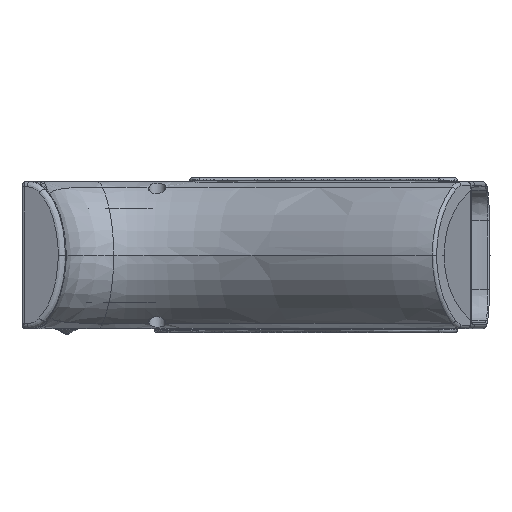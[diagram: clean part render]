
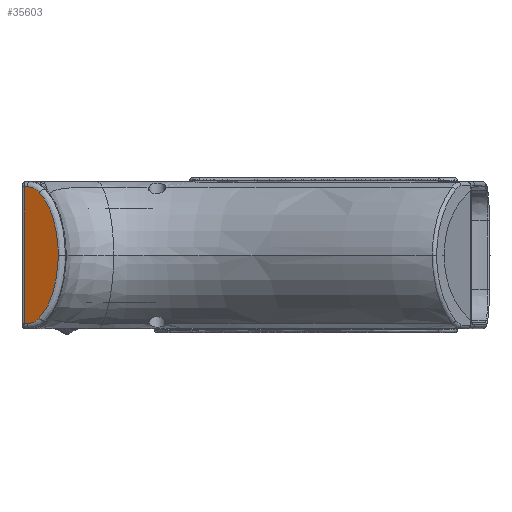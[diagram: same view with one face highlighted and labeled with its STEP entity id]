
A CAD part, left-side view. The second image highlights one B-rep face of the part: STEP entity #35603.
In plain terms, the highlighted planar face has unit normal (-0.906, 0.423, 0).
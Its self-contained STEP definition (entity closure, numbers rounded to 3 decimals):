
#2019=PLANE('',#37724);
#3836=FACE_OUTER_BOUND('',#5931,.T.);
#5931=EDGE_LOOP('',(#24339,#24340,#24341,#24342,#24343,#24344,#24345));
#8334=LINE('',#45406,#11125);
#8445=LINE('',#54969,#11236);
#8446=LINE('',#55000,#11237);
#11125=VECTOR('',#39023,1.);
#11236=VECTOR('',#39260,10.);
#11237=VECTOR('',#39261,1.);
#13998=B_SPLINE_CURVE_WITH_KNOTS('',3,(#54913,#54914,#54915,#54916,#54917,
#54918,#54919,#54920,#54921,#54922,#54923,#54924,#54925,#54926,#54927,#54928,
#54929,#54930,#54931,#54932,#54933,#54934,#54935,#54936,#54937),
 .UNSPECIFIED.,.F.,.F.,(4,2,2,2,2,2,2,2,2,1,2,2,4),(0.003,
0.144,0.288,0.431,0.573,0.714,
0.855,0.996,1.135,1.188,1.241,
1.293,1.332),.UNSPECIFIED.);
#13999=B_SPLINE_CURVE_WITH_KNOTS('',3,(#54963,#54964,#54965,#54966),
 .UNSPECIFIED.,.F.,.F.,(4,4),(-0.284,0.),.UNSPECIFIED.);
#14000=B_SPLINE_CURVE_WITH_KNOTS('',3,(#54971,#54972,#54973,#54974,#54975,
#54976,#54977,#54978,#54979,#54980,#54981,#54982,#54983,#54984,#54985,#54986,
#54987,#54988,#54989,#54990,#54991,#54992,#54993,#54994),.UNSPECIFIED.,
 .F.,.F.,(4,2,2,2,2,2,2,2,2,2,2,4),(0.197,0.236,0.287,
0.394,0.533,0.673,0.813,0.954,
1.096,1.239,1.383,1.523),
 .UNSPECIFIED.);
#14001=B_SPLINE_CURVE_WITH_KNOTS('',3,(#54996,#54997,#54998,#54999),
 .UNSPECIFIED.,.F.,.F.,(4,4),(-0.284,0.),.UNSPECIFIED.);
#14728=VERTEX_POINT('',#45401);
#14729=VERTEX_POINT('',#45404);
#14905=VERTEX_POINT('',#54460);
#14906=VERTEX_POINT('',#54912);
#14907=VERTEX_POINT('',#54968);
#14908=VERTEX_POINT('',#54970);
#14909=VERTEX_POINT('',#54995);
#18337=EDGE_CURVE('',#14729,#14728,#8334,.T.);
#18559=EDGE_CURVE('',#14905,#14906,#13998,.T.);
#18561=EDGE_CURVE('',#14906,#14729,#13999,.T.);
#18562=EDGE_CURVE('',#14728,#14907,#8445,.T.);
#18563=EDGE_CURVE('',#14908,#14905,#14000,.T.);
#18564=EDGE_CURVE('',#14909,#14908,#14001,.T.);
#18565=EDGE_CURVE('',#14907,#14909,#8446,.T.);
#24339=ORIENTED_EDGE('',*,*,#18562,.F.);
#24340=ORIENTED_EDGE('',*,*,#18337,.F.);
#24341=ORIENTED_EDGE('',*,*,#18561,.F.);
#24342=ORIENTED_EDGE('',*,*,#18559,.F.);
#24343=ORIENTED_EDGE('',*,*,#18563,.F.);
#24344=ORIENTED_EDGE('',*,*,#18564,.F.);
#24345=ORIENTED_EDGE('',*,*,#18565,.F.);
#35603=ADVANCED_FACE('',(#3836),#2019,.F.);
#37724=AXIS2_PLACEMENT_3D('',#54967,#39258,#39259);
#39023=DIRECTION('',(0.423,0.906,0.));
#39258=DIRECTION('center_axis',(0.906,-0.423,0.));
#39259=DIRECTION('ref_axis',(0.423,0.906,0.));
#39260=DIRECTION('',(0.,0.,1.));
#39261=DIRECTION('',(-0.423,-0.906,0.));
#45401=CARTESIAN_POINT('',(-0.852,-1.404,-13.4));
#45404=CARTESIAN_POINT('',(-1.16,-2.065,-13.4));
#45406=CARTESIAN_POINT('',(-5.081,-10.474,-13.4));
#54460=CARTESIAN_POINT('',(-3.998,-8.151,0.));
#54912=CARTESIAN_POINT('',(-2.228,-4.355,-12.302));
#54913=CARTESIAN_POINT('Ctrl Pts',(-3.998,-8.151,
0.));
#54914=CARTESIAN_POINT('Ctrl Pts',(-3.99,-8.134,
-0.469));
#54915=CARTESIAN_POINT('Ctrl Pts',(-3.979,-8.11,-0.938));
#54916=CARTESIAN_POINT('Ctrl Pts',(-3.948,-8.045,-1.883));
#54917=CARTESIAN_POINT('Ctrl Pts',(-3.929,-8.003,-2.36));
#54918=CARTESIAN_POINT('Ctrl Pts',(-3.88,-7.898,-3.311));
#54919=CARTESIAN_POINT('Ctrl Pts',(-3.851,-7.836,-3.785));
#54920=CARTESIAN_POINT('Ctrl Pts',(-3.782,-7.688,-4.724));
#54921=CARTESIAN_POINT('Ctrl Pts',(-3.742,-7.603,-5.191));
#54922=CARTESIAN_POINT('Ctrl Pts',(-3.649,-7.404,-6.114));
#54923=CARTESIAN_POINT('Ctrl Pts',(-3.597,-7.291,-6.57));
#54924=CARTESIAN_POINT('Ctrl Pts',(-3.476,-7.032,-7.47));
#54925=CARTESIAN_POINT('Ctrl Pts',(-3.409,-6.887,-7.913));
#54926=CARTESIAN_POINT('Ctrl Pts',(-3.256,-6.56,-8.782));
#54927=CARTESIAN_POINT('Ctrl Pts',(-3.171,-6.378,-9.207));
#54928=CARTESIAN_POINT('Ctrl Pts',(-2.982,-5.973,-10.028));
#54929=CARTESIAN_POINT('Ctrl Pts',(-2.878,-5.75,-10.423));
#54930=CARTESIAN_POINT('Ctrl Pts',(-2.72,-5.412,-10.944));
#54931=CARTESIAN_POINT('Ctrl Pts',(-2.63,-5.218,-11.226));
#54932=CARTESIAN_POINT('Ctrl Pts',(-2.533,-5.01,-11.496));
#54933=CARTESIAN_POINT('Ctrl Pts',(-2.435,-4.799,-11.756));
#54934=CARTESIAN_POINT('Ctrl Pts',(-2.387,-4.696,-11.883));
#54935=CARTESIAN_POINT('Ctrl Pts',(-2.301,-4.513,-12.108));
#54936=CARTESIAN_POINT('Ctrl Pts',(-2.264,-4.434,-12.205));
#54937=CARTESIAN_POINT('Ctrl Pts',(-2.228,-4.355,-12.302));
#54963=CARTESIAN_POINT('Ctrl Pts',(-2.228,-4.355,-12.302));
#54964=CARTESIAN_POINT('Ctrl Pts',(-1.961,-3.783,-13.006));
#54965=CARTESIAN_POINT('Ctrl Pts',(-1.559,-2.922,-13.4));
#54966=CARTESIAN_POINT('Ctrl Pts',(-1.16,-2.065,-13.4));
#54967=CARTESIAN_POINT('Origin',(-10.,-21.023,-17.642));
#54968=CARTESIAN_POINT('',(-0.852,-1.404,13.4));
#54969=CARTESIAN_POINT('',(-0.852,-1.404,0.036));
#54970=CARTESIAN_POINT('',(-2.228,-4.355,12.302));
#54971=CARTESIAN_POINT('Ctrl Pts',(-2.228,-4.355,12.302));
#54972=CARTESIAN_POINT('Ctrl Pts',(-2.264,-4.434,12.205));
#54973=CARTESIAN_POINT('Ctrl Pts',(-2.301,-4.513,12.108));
#54974=CARTESIAN_POINT('Ctrl Pts',(-2.387,-4.696,11.883));
#54975=CARTESIAN_POINT('Ctrl Pts',(-2.435,-4.799,11.756));
#54976=CARTESIAN_POINT('Ctrl Pts',(-2.583,-5.117,11.365));
#54977=CARTESIAN_POINT('Ctrl Pts',(-2.677,-5.318,11.088));
#54978=CARTESIAN_POINT('Ctrl Pts',(-2.878,-5.75,10.423));
#54979=CARTESIAN_POINT('Ctrl Pts',(-2.982,-5.973,10.028));
#54980=CARTESIAN_POINT('Ctrl Pts',(-3.171,-6.377,9.208));
#54981=CARTESIAN_POINT('Ctrl Pts',(-3.256,-6.559,8.783));
#54982=CARTESIAN_POINT('Ctrl Pts',(-3.408,-6.887,7.914));
#54983=CARTESIAN_POINT('Ctrl Pts',(-3.476,-7.033,7.47));
#54984=CARTESIAN_POINT('Ctrl Pts',(-3.597,-7.292,6.568));
#54985=CARTESIAN_POINT('Ctrl Pts',(-3.65,-7.405,6.111));
#54986=CARTESIAN_POINT('Ctrl Pts',(-3.742,-7.603,5.191));
#54987=CARTESIAN_POINT('Ctrl Pts',(-3.782,-7.688,4.724));
#54988=CARTESIAN_POINT('Ctrl Pts',(-3.851,-7.836,3.785));
#54989=CARTESIAN_POINT('Ctrl Pts',(-3.88,-7.898,3.312));
#54990=CARTESIAN_POINT('Ctrl Pts',(-3.929,-8.003,2.361));
#54991=CARTESIAN_POINT('Ctrl Pts',(-3.948,-8.045,1.884));
#54992=CARTESIAN_POINT('Ctrl Pts',(-3.979,-8.11,0.937));
#54993=CARTESIAN_POINT('Ctrl Pts',(-3.99,-8.134,0.468));
#54994=CARTESIAN_POINT('Ctrl Pts',(-3.998,-8.151,0.));
#54995=CARTESIAN_POINT('',(-1.16,-2.065,13.4));
#54996=CARTESIAN_POINT('Ctrl Pts',(-1.16,-2.065,13.4));
#54997=CARTESIAN_POINT('Ctrl Pts',(-1.559,-2.922,13.4));
#54998=CARTESIAN_POINT('Ctrl Pts',(-1.961,-3.783,13.006));
#54999=CARTESIAN_POINT('Ctrl Pts',(-2.228,-4.355,12.302));
#55000=CARTESIAN_POINT('',(-5.758,-11.925,13.4));
